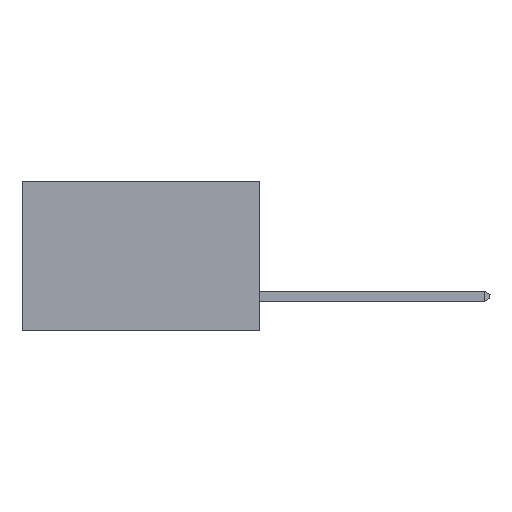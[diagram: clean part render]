
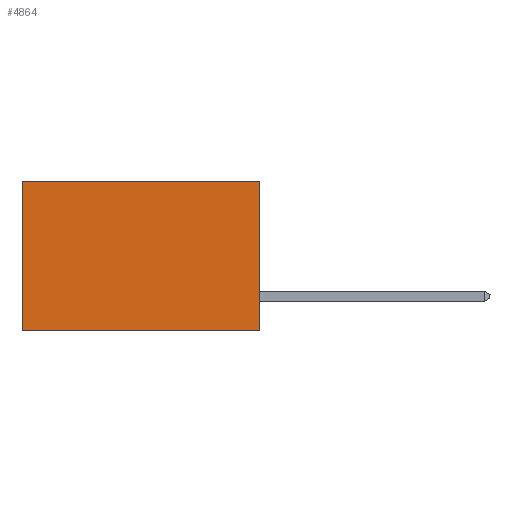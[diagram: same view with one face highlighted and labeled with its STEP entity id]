
A CAD part, left-side view. The second image highlights one B-rep face of the part: STEP entity #4864.
In plain terms, the highlighted planar face has unit normal (-1, 0, 0).
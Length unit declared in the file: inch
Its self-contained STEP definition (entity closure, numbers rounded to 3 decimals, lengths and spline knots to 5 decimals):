
#291 = LINE ( 'NONE', #8506, #2730 ) ;
#921 = DIRECTION ( 'NONE',  ( 0., 1., 0. ) ) ;
#939 = CARTESIAN_POINT ( 'NONE',  ( 0.277, 0., 0. ) ) ;
#1401 = DIRECTION ( 'NONE',  ( 0., 1., 0. ) ) ;
#1428 = EDGE_CURVE ( 'NONE', #1994, #2501, #291, .T. ) ;
#1506 = CARTESIAN_POINT ( 'NONE',  ( 0.277, 0., 0. ) ) ;
#1897 = EDGE_CURVE ( 'NONE', #6337, #1994, #4848, .T. ) ;
#1994 = VERTEX_POINT ( 'NONE', #6342 ) ;
#2501 = VERTEX_POINT ( 'NONE', #8426 ) ;
#2539 = EDGE_LOOP ( 'NONE', ( #5011, #5490, #7944, #2794 ) ) ;
#2719 = VECTOR ( 'NONE', #4793, 39.37008 ) ;
#2730 = VECTOR ( 'NONE', #1401, 39.37008 ) ;
#2794 = ORIENTED_EDGE ( 'NONE', *, *, #7894, .T. ) ;
#3060 = LINE ( 'NONE', #939, #6948 ) ;
#3147 = CARTESIAN_POINT ( 'NONE',  ( 0.277, 0., -0.37 ) ) ;
#3421 = DIRECTION ( 'NONE',  ( 0., 0., -1. ) ) ;
#3546 = CARTESIAN_POINT ( 'NONE',  ( 0.277, 0.59, -0.37 ) ) ;
#4356 = VERTEX_POINT ( 'NONE', #5116 ) ;
#4793 = DIRECTION ( 'NONE',  ( 0., 0., -1. ) ) ;
#4848 = LINE ( 'NONE', #3147, #2719 ) ;
#4864 = ADVANCED_FACE ( 'NONE', ( #8169 ), #6512, .F. ) ;
#5011 = ORIENTED_EDGE ( 'NONE', *, *, #6844, .T. ) ;
#5116 = CARTESIAN_POINT ( 'NONE',  ( 0.277, 0.59, 0. ) ) ;
#5490 = ORIENTED_EDGE ( 'NONE', *, *, #1428, .F. ) ;
#5958 = DIRECTION ( 'NONE',  ( 0., 0., -1. ) ) ;
#6024 = DIRECTION ( 'NONE',  ( 1., 0., 0. ) ) ;
#6290 = VECTOR ( 'NONE', #3421, 39.37008 ) ;
#6337 = VERTEX_POINT ( 'NONE', #1506 ) ;
#6342 = CARTESIAN_POINT ( 'NONE',  ( 0.277, 0., -0.37 ) ) ;
#6491 = CARTESIAN_POINT ( 'NONE',  ( 0.277, 0., -0.37 ) ) ;
#6512 = PLANE ( 'NONE',  #7628 ) ;
#6844 = EDGE_CURVE ( 'NONE', #4356, #2501, #8216, .T. ) ;
#6948 = VECTOR ( 'NONE', #921, 39.37008 ) ;
#7628 = AXIS2_PLACEMENT_3D ( 'NONE', #6491, #6024, #5958 ) ;
#7894 = EDGE_CURVE ( 'NONE', #6337, #4356, #3060, .T. ) ;
#7944 = ORIENTED_EDGE ( 'NONE', *, *, #1897, .F. ) ;
#8169 = FACE_OUTER_BOUND ( 'NONE', #2539, .T. ) ;
#8216 = LINE ( 'NONE', #3546, #6290 ) ;
#8426 = CARTESIAN_POINT ( 'NONE',  ( 0.277, 0.59, -0.37 ) ) ;
#8506 = CARTESIAN_POINT ( 'NONE',  ( 0.277, 0., -0.37 ) ) ;
